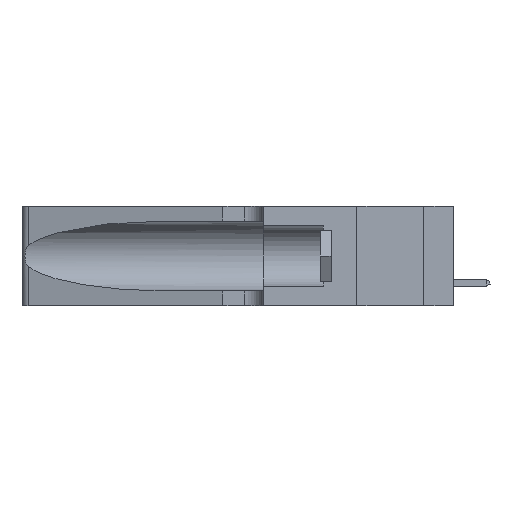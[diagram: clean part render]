
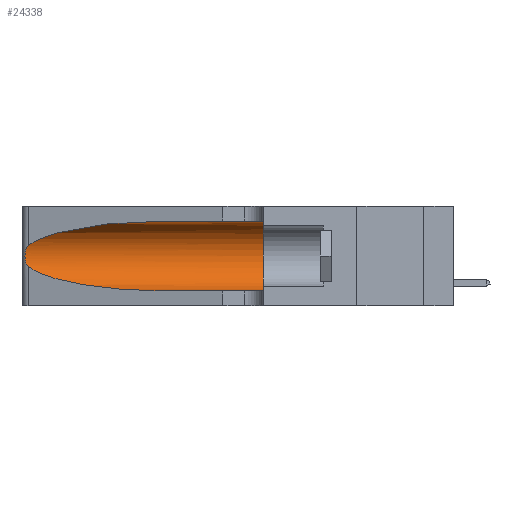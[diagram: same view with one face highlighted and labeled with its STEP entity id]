
A CAD part, left-side view. The second image highlights one B-rep face of the part: STEP entity #24338.
In plain terms, the highlighted cylindrical face has radius 3.308 mm (diameter 6.617 mm), a partial arc.
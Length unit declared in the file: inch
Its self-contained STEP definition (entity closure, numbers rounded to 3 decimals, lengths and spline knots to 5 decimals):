
#113 = VERTEX_POINT ( 'NONE', #32655 ) ;
#352 = ORIENTED_EDGE ( 'NONE', *, *, #4469, .T. ) ;
#1978 = CARTESIAN_POINT ( 'NONE',  ( 0.26018, 1.23835, 0.19895 ) ) ;
#2528 = ORIENTED_EDGE ( 'NONE', *, *, #33616, .F. ) ;
#3875 = CARTESIAN_POINT ( 'NONE',  ( 0.1305, 0.72297, 0.05475 ) ) ;
#4469 = EDGE_CURVE ( 'NONE', #14052, #11290, #22312, .T. ) ;
#4742 = CARTESIAN_POINT ( 'NONE',  ( 0.25789, 1.23486, 0.15765 ) ) ;
#4856 = CARTESIAN_POINT ( 'NONE',  ( 0.25639, 1.23186, 0.15144 ) ) ;
#6135 = CARTESIAN_POINT ( 'NONE',  ( 0.25487, 1.22718, 0.22369 ) ) ;
#6288 = CARTESIAN_POINT ( 'NONE',  ( 0.1305, 0.72297, 0.05475 ) ) ;
#6753 = EDGE_CURVE ( 'NONE', #14052, #113, #25164, .T. ) ;
#7056 = CARTESIAN_POINT ( 'NONE',  ( 0.25487, 1.22718, 0.22369 ) ) ;
#7307 = CARTESIAN_POINT ( 'NONE',  ( 0.25787, 1.23484, 0.2124 ) ) ;
#9230 = DIRECTION ( 'NONE',  ( 0., 1., 0. ) ) ;
#10027 = CARTESIAN_POINT ( 'NONE',  ( 0.25854, 1.2359, 0.20912 ) ) ;
#10520 = CARTESIAN_POINT ( 'NONE',  ( 0.1305, 0.72297, 0.31525 ) ) ;
#10529 = ORIENTED_EDGE ( 'NONE', *, *, #6753, .F. ) ;
#10749 = VECTOR ( 'NONE', #29555, 39.37008 ) ;
#10938 = VERTEX_POINT ( 'NONE', #6288 ) ;
#11082 = CARTESIAN_POINT ( 'NONE',  ( 0.2373, 1.15595, 0.28018 ) ) ;
#11290 = VERTEX_POINT ( 'NONE', #6135 ) ;
#11368 = CIRCLE ( 'NONE', #25582, 0.13025 ) ;
#11903 = CARTESIAN_POINT ( 'NONE',  ( 0.25487, 1.22718, 0.14631 ) ) ;
#12371 = EDGE_CURVE ( 'NONE', #10938, #19526, #16970, .T. ) ;
#13258 = CARTESIAN_POINT ( 'NONE',  ( 0.25487, 1.22718, 0.14631 ) ) ;
#13339 = CARTESIAN_POINT ( 'NONE',  ( 0.26017, 1.23833, 0.17102 ) ) ;
#13539 = DIRECTION ( 'NONE',  ( 0., -1., 0. ) ) ;
#13700 = CARTESIAN_POINT ( 'NONE',  ( 0.18966, 0.96281, 0.31525 ) ) ;
#13733 = EDGE_LOOP ( 'NONE', ( #352, #17471, #21988, #22306, #2528, #10529 ) ) ;
#14052 = VERTEX_POINT ( 'NONE', #10520 ) ;
#14610 = CARTESIAN_POINT ( 'NONE',  ( 0.2373, 1.15595, 0.08982 ) ) ;
#14941 = DIRECTION ( 'NONE',  ( 0., 0., -1. ) ) ;
#15411 = EDGE_CURVE ( 'NONE', #33968, #10938, #26080, .T. ) ;
#16260 = CARTESIAN_POINT ( 'NONE',  ( 0.25487, 1.22718, 0.22369 ) ) ;
#16599 = CARTESIAN_POINT ( 'NONE',  ( 0.1305, 0.72297, 0.31525 ) ) ;
#16970 = LINE ( 'NONE', #26743, #34891 ) ;
#17471 = ORIENTED_EDGE ( 'NONE', *, *, #20283, .T. ) ;
#17797 = CARTESIAN_POINT ( 'NONE',  ( 0.1305, 0.35, 0.05475 ) ) ;
#19526 = VERTEX_POINT ( 'NONE', #17797 ) ;
#20283 = EDGE_CURVE ( 'NONE', #11290, #33968, #29342, .T. ) ;
#20719 = FACE_OUTER_BOUND ( 'NONE', #13733, .T. ) ;
#20941 = CARTESIAN_POINT ( 'NONE',  ( 0.25856, 1.23593, 0.16098 ) ) ;
#21443 = AXIS2_PLACEMENT_3D ( 'NONE', #25258, #31104, #14941 ) ;
#21988 = ORIENTED_EDGE ( 'NONE', *, *, #15411, .T. ) ;
#22306 = ORIENTED_EDGE ( 'NONE', *, *, #12371, .T. ) ;
#22312 =( BOUNDED_CURVE ( )  B_SPLINE_CURVE ( 3, ( #16599, #13700, #11082, #16260 ),
 .UNSPECIFIED., .F., .T. ) 
 B_SPLINE_CURVE_WITH_KNOTS ( ( 4, 4 ),
 ( 1.5708, 2.84003 ),
 .UNSPECIFIED. ) 
 CURVE ( )  GEOMETRIC_REPRESENTATION_ITEM ( )  RATIONAL_B_SPLINE_CURVE ( ( 1., 0.87, 0.87, 1. ) ) 
 REPRESENTATION_ITEM ( '' )  );
#23047 = CARTESIAN_POINT ( 'NONE',  ( 0.18966, 0.96281, 0.05475 ) ) ;
#23538 = CARTESIAN_POINT ( 'NONE',  ( 0.25639, 1.23184, 0.21858 ) ) ;
#23657 = CARTESIAN_POINT ( 'NONE',  ( 0.25555, 1.22993, 0.14849 ) ) ;
#24338 = ADVANCED_FACE ( 'NONE', ( #20719 ), #27089, .F. ) ;
#25164 = LINE ( 'NONE', #32014, #10749 ) ;
#25258 = CARTESIAN_POINT ( 'NONE',  ( 0.1305, 1.61858, 0.185 ) ) ;
#25582 = AXIS2_PLACEMENT_3D ( 'NONE', #30945, #9230, #33692 ) ;
#26080 =( BOUNDED_CURVE ( )  B_SPLINE_CURVE ( 3, ( #11903, #14610, #23047, #3875 ),
 .UNSPECIFIED., .F., .F. ) 
 B_SPLINE_CURVE_WITH_KNOTS ( ( 4, 4 ),
 ( 3.44316, 4.71239 ),
 .UNSPECIFIED. ) 
 CURVE ( )  GEOMETRIC_REPRESENTATION_ITEM ( )  RATIONAL_B_SPLINE_CURVE ( ( 1., 0.87, 0.87, 1. ) ) 
 REPRESENTATION_ITEM ( '' )  );
#26743 = CARTESIAN_POINT ( 'NONE',  ( 0.1305, 1.61858, 0.05475 ) ) ;
#26876 = CARTESIAN_POINT ( 'NONE',  ( 0.26075, 1.23896, 0.178 ) ) ;
#27089 = CYLINDRICAL_SURFACE ( 'NONE', #21443, 0.13025 ) ;
#29141 = CARTESIAN_POINT ( 'NONE',  ( 0.25487, 1.22718, 0.14631 ) ) ;
#29342 = B_SPLINE_CURVE_WITH_KNOTS ( 'NONE', 3,
 ( #7056, #34012, #23538, #7307, #10027, #1978, #34920, #26876, #13339, #20941, #4742, #4856, #23657, #29141 ),
 .UNSPECIFIED., .F., .F.,
 ( 4, 2, 2, 2, 2, 2, 4 ),
 ( 0., 0.00027, 0.00053, 0.00107, 0.0016, 0.00187, 0.00214 ),
 .UNSPECIFIED. ) ;
#29555 = DIRECTION ( 'NONE',  ( 0., -1., 0. ) ) ;
#30945 = CARTESIAN_POINT ( 'NONE',  ( 0.1305, 0.35, 0.185 ) ) ;
#31104 = DIRECTION ( 'NONE',  ( 0., -1., 0. ) ) ;
#32014 = CARTESIAN_POINT ( 'NONE',  ( 0.1305, 1.61858, 0.31525 ) ) ;
#32655 = CARTESIAN_POINT ( 'NONE',  ( 0.1305, 0.35, 0.31525 ) ) ;
#33616 = EDGE_CURVE ( 'NONE', #113, #19526, #11368, .T. ) ;
#33692 = DIRECTION ( 'NONE',  ( 0., 0., 1. ) ) ;
#33968 = VERTEX_POINT ( 'NONE', #13258 ) ;
#34012 = CARTESIAN_POINT ( 'NONE',  ( 0.25555, 1.22994, 0.2215 ) ) ;
#34891 = VECTOR ( 'NONE', #13539, 39.37008 ) ;
#34920 = CARTESIAN_POINT ( 'NONE',  ( 0.26075, 1.23896, 0.19203 ) ) ;
